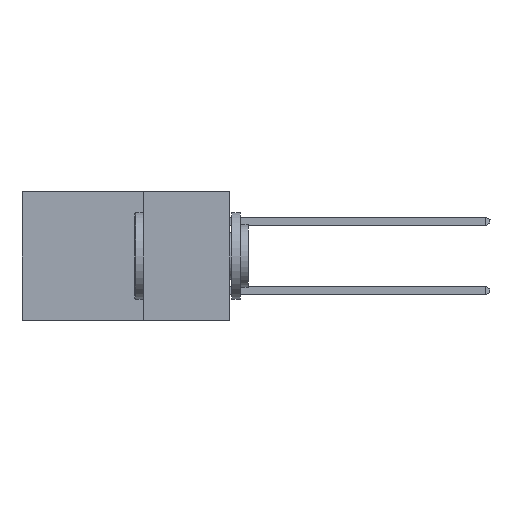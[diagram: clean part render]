
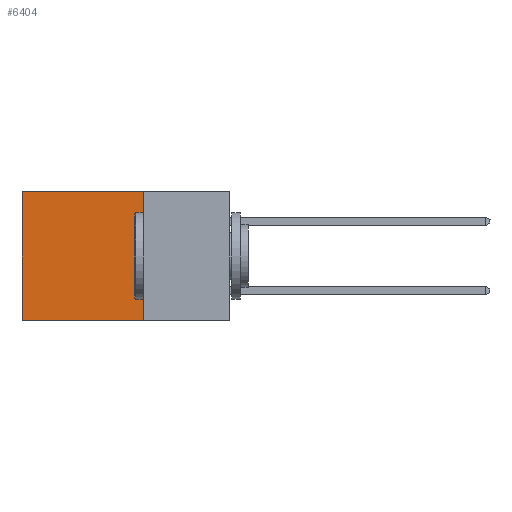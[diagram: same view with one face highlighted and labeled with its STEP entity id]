
A CAD part, left-side view. The second image highlights one B-rep face of the part: STEP entity #6404.
In plain terms, the highlighted planar face has unit normal (-1, 0, 0).
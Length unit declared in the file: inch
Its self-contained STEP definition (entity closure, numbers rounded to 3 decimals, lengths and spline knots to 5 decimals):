
#713 = ORIENTED_EDGE ( 'NONE', *, *, #2778, .F. ) ;
#953 = CARTESIAN_POINT ( 'NONE',  ( 0.2615, 0.6, -0.37 ) ) ;
#1505 = EDGE_LOOP ( 'NONE', ( #2546, #8478, #713, #2544 ) ) ;
#2089 = EDGE_CURVE ( 'NONE', #11467, #9009, #2280, .T. ) ;
#2280 = LINE ( 'NONE', #6049, #6040 ) ;
#2544 = ORIENTED_EDGE ( 'NONE', *, *, #10040, .T. ) ;
#2546 = ORIENTED_EDGE ( 'NONE', *, *, #4068, .T. ) ;
#2723 = VERTEX_POINT ( 'NONE', #12255 ) ;
#2769 = VERTEX_POINT ( 'NONE', #10401 ) ;
#2778 = EDGE_CURVE ( 'NONE', #2769, #11467, #11401, .T. ) ;
#2812 = DIRECTION ( 'NONE',  ( 0., 0., -1. ) ) ;
#3146 = CARTESIAN_POINT ( 'NONE',  ( 0.2615, 0.25, -0.37 ) ) ;
#3446 = LINE ( 'NONE', #7228, #3768 ) ;
#3709 = CARTESIAN_POINT ( 'NONE',  ( 0.2615, 0.25, -0.37 ) ) ;
#3768 = VECTOR ( 'NONE', #7293, 39.37008 ) ;
#4068 = EDGE_CURVE ( 'NONE', #2723, #9009, #9393, .T. ) ;
#5133 = PLANE ( 'NONE',  #9852 ) ;
#5152 = CARTESIAN_POINT ( 'NONE',  ( 0.2615, 0.6, -0.37 ) ) ;
#5728 = DIRECTION ( 'NONE',  ( 0., 0., -1. ) ) ;
#5844 = VECTOR ( 'NONE', #5728, 39.37008 ) ;
#6040 = VECTOR ( 'NONE', #9850, 39.37008 ) ;
#6049 = CARTESIAN_POINT ( 'NONE',  ( 0.2615, 0.25, -0.37 ) ) ;
#6404 = ADVANCED_FACE ( 'NONE', ( #11673 ), #5133, .F. ) ;
#6652 = CARTESIAN_POINT ( 'NONE',  ( 0.2615, 0.25, -0.37 ) ) ;
#7228 = CARTESIAN_POINT ( 'NONE',  ( 0.2615, 0.25, 0. ) ) ;
#7293 = DIRECTION ( 'NONE',  ( 0., 1., 0. ) ) ;
#7993 = DIRECTION ( 'NONE',  ( 0., 0., -1. ) ) ;
#8478 = ORIENTED_EDGE ( 'NONE', *, *, #2089, .F. ) ;
#8926 = DIRECTION ( 'NONE',  ( 1., 0., 0. ) ) ;
#9009 = VERTEX_POINT ( 'NONE', #5152 ) ;
#9393 = LINE ( 'NONE', #953, #10452 ) ;
#9850 = DIRECTION ( 'NONE',  ( 0., 1., 0. ) ) ;
#9852 = AXIS2_PLACEMENT_3D ( 'NONE', #3146, #8926, #7993 ) ;
#10040 = EDGE_CURVE ( 'NONE', #2769, #2723, #3446, .T. ) ;
#10401 = CARTESIAN_POINT ( 'NONE',  ( 0.2615, 0.25, 0. ) ) ;
#10452 = VECTOR ( 'NONE', #2812, 39.37008 ) ;
#11401 = LINE ( 'NONE', #6652, #5844 ) ;
#11467 = VERTEX_POINT ( 'NONE', #3709 ) ;
#11673 = FACE_OUTER_BOUND ( 'NONE', #1505, .T. ) ;
#12255 = CARTESIAN_POINT ( 'NONE',  ( 0.2615, 0.6, 0. ) ) ;
